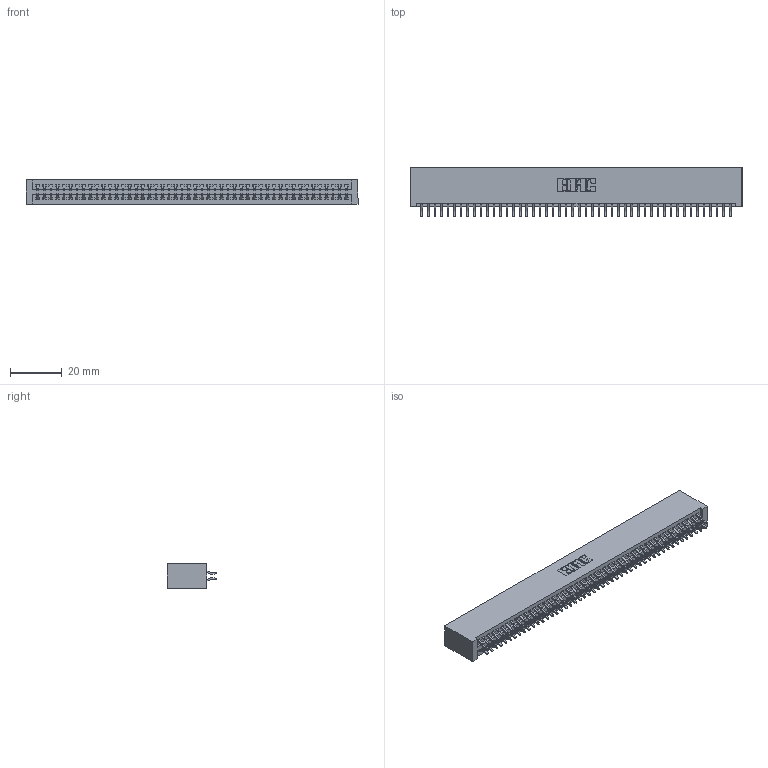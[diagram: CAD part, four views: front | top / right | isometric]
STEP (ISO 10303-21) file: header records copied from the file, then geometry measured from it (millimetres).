
FILE_DESCRIPTION (( 'STEP AP203' ), '1' );
FILE_NAME ('395-096-556-201.STEP', '2018-11-29T16:47:42', ( '' ), ( '' ), 'SwSTEP 2.0', 'SolidWorks 2016', '' );
FILE_SCHEMA (( 'CONFIG_CONTROL_DESIGN' ));
Length unit declared in the file: inch
Products named in the file (3): 395-096-556-201; 345-292-001_556 Tail; 345 Part_No Mounting Lugs
Assembly tree (97 placements, depth 2):
  395-096-556-201
    345 Part_No Mounting Lugs
    345-292-001_556 Tail  x96
Bounding box: 128.52 x 19.24 x 9.4 mm (x, y, z)
Volume: 13152.8 mm3; surface area: 19777.4 mm2
Topology: 97 solids, 97 shells, 5494 faces, 16349 edges, 10770 vertices
Faces by surface type: plane 3628, cylinder 1866
Entity records: 36797 total; most frequent: CARTESIAN_POINT 6176, ORIENTED_EDGE 6098, DIRECTION 5421, EDGE_CURVE 3049, VECTOR 2725, LINE 2725, VERTEX_POINT 2030, AXIS2_PLACEMENT_3D 1348
